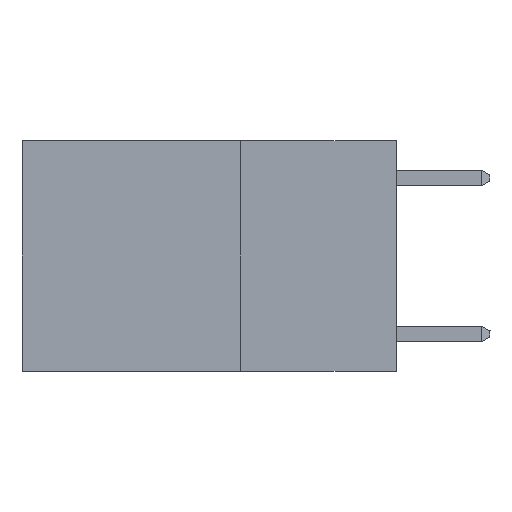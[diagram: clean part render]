
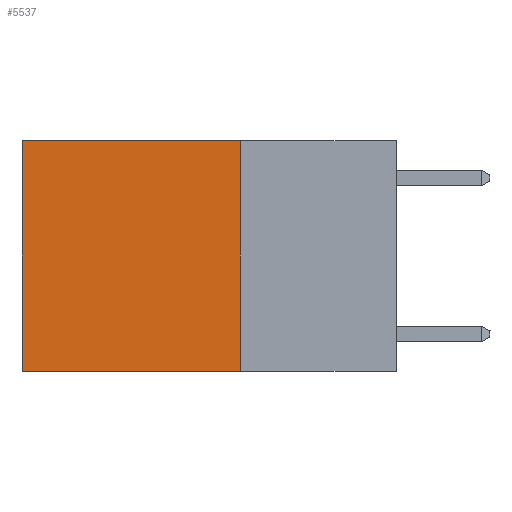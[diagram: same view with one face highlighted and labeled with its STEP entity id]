
A CAD part, left-side view. The second image highlights one B-rep face of the part: STEP entity #5537.
In plain terms, the highlighted planar face has unit normal (-1, 0, 0).
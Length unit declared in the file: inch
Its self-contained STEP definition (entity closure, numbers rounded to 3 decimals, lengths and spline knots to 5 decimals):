
#383 = VERTEX_POINT ( 'NONE', #2287 ) ;
#513 = VECTOR ( 'NONE', #544, 39.37008 ) ;
#544 = DIRECTION ( 'NONE',  ( 0., 1., 0. ) ) ;
#627 = CARTESIAN_POINT ( 'NONE',  ( 0.2625, 0.25, 0. ) ) ;
#797 = VECTOR ( 'NONE', #5958, 39.37008 ) ;
#904 = FACE_OUTER_BOUND ( 'NONE', #10832, .T. ) ;
#1529 = VECTOR ( 'NONE', #6691, 39.37008 ) ;
#2287 = CARTESIAN_POINT ( 'NONE',  ( 0.2625, 0.6, 0. ) ) ;
#3052 = ORIENTED_EDGE ( 'NONE', *, *, #9567, .T. ) ;
#3176 = DIRECTION ( 'NONE',  ( 0., 0., -1. ) ) ;
#4103 = VERTEX_POINT ( 'NONE', #6397 ) ;
#4456 = LINE ( 'NONE', #9865, #797 ) ;
#5054 = EDGE_CURVE ( 'NONE', #9790, #4103, #6789, .T. ) ;
#5118 = DIRECTION ( 'NONE',  ( 1., 0., 0. ) ) ;
#5334 = CARTESIAN_POINT ( 'NONE',  ( 0.2625, 0.25, -0.37 ) ) ;
#5390 = VECTOR ( 'NONE', #12806, 39.37008 ) ;
#5505 = CARTESIAN_POINT ( 'NONE',  ( 0.2625, 0.25, -0.37 ) ) ;
#5537 = ADVANCED_FACE ( 'NONE', ( #904 ), #6260, .F. ) ;
#5958 = DIRECTION ( 'NONE',  ( 0., 0., -1. ) ) ;
#6260 = PLANE ( 'NONE',  #6524 ) ;
#6397 = CARTESIAN_POINT ( 'NONE',  ( 0.2625, 0.6, -0.37 ) ) ;
#6524 = AXIS2_PLACEMENT_3D ( 'NONE', #8097, #5118, #3176 ) ;
#6691 = DIRECTION ( 'NONE',  ( 0., 1., 0. ) ) ;
#6789 = LINE ( 'NONE', #5505, #1529 ) ;
#7284 = LINE ( 'NONE', #627, #5390 ) ;
#7496 = ORIENTED_EDGE ( 'NONE', *, *, #5054, .F. ) ;
#7623 = ORIENTED_EDGE ( 'NONE', *, *, #10320, .T. ) ;
#8097 = CARTESIAN_POINT ( 'NONE',  ( 0.2625, 0.25, 0. ) ) ;
#8607 = CARTESIAN_POINT ( 'NONE',  ( 0.2625, 0.25, 0. ) ) ;
#9567 = EDGE_CURVE ( 'NONE', #383, #4103, #4456, .T. ) ;
#9790 = VERTEX_POINT ( 'NONE', #5334 ) ;
#9865 = CARTESIAN_POINT ( 'NONE',  ( 0.2625, 0.6, 0. ) ) ;
#10320 = EDGE_CURVE ( 'NONE', #12401, #383, #11267, .T. ) ;
#10562 = ORIENTED_EDGE ( 'NONE', *, *, #12856, .F. ) ;
#10832 = EDGE_LOOP ( 'NONE', ( #3052, #7496, #10562, #7623 ) ) ;
#11267 = LINE ( 'NONE', #8607, #513 ) ;
#11913 = CARTESIAN_POINT ( 'NONE',  ( 0.2625, 0.25, 0. ) ) ;
#12401 = VERTEX_POINT ( 'NONE', #11913 ) ;
#12806 = DIRECTION ( 'NONE',  ( 0., 0., -1. ) ) ;
#12856 = EDGE_CURVE ( 'NONE', #12401, #9790, #7284, .T. ) ;
